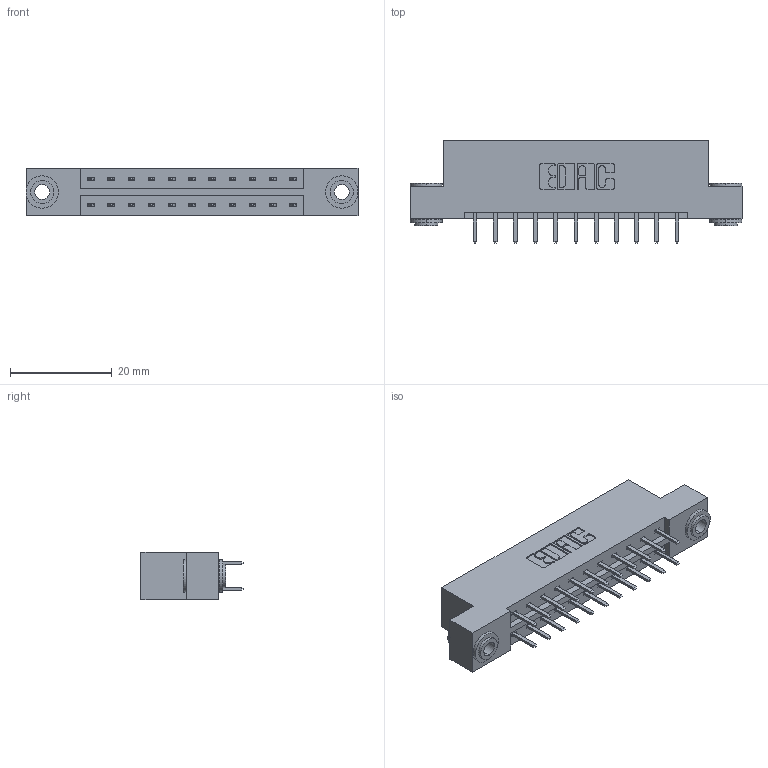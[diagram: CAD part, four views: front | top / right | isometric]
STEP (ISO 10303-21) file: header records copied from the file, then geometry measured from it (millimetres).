
FILE_DESCRIPTION (( 'STEP AP203' ), '1' );
FILE_NAME ('833-022-520-203.STEP', '2020-06-01T15:57:52', ( '' ), ( '' ), 'SwSTEP 2.0', 'SolidWorks 2020', '' );
FILE_SCHEMA (( 'CONFIG_CONTROL_DESIGN' ));
Length unit declared in the file: inch
Products named in the file (4): 345-292-001_345-293-120; 833 Part_Flush - .156 Dia - TH; 345-250-002_345-250-002-102; 833-022-520-203
Assembly tree (25 placements, depth 2):
  833-022-520-203
    833 Part_Flush - .156 Dia - TH
    345-292-001_345-293-120  x22
    345-250-002_345-250-002-102  x2
Bounding box: 65.13 x 20.02 x 9.4 mm (x, y, z)
Volume: 6368.8 mm3; surface area: 7391.6 mm2
Topology: 25 solids, 25 shells, 1384 faces, 3973 edges, 2586 vertices
Faces by surface type: plane 916, cylinder 460, cone 8
Entity records: 11850 total; most frequent: CARTESIAN_POINT 1989, ORIENTED_EDGE 1906, DIRECTION 1775, EDGE_CURVE 953, LINE 797, VECTOR 797, VERTEX_POINT 630, AXIS2_PLACEMENT_3D 489
